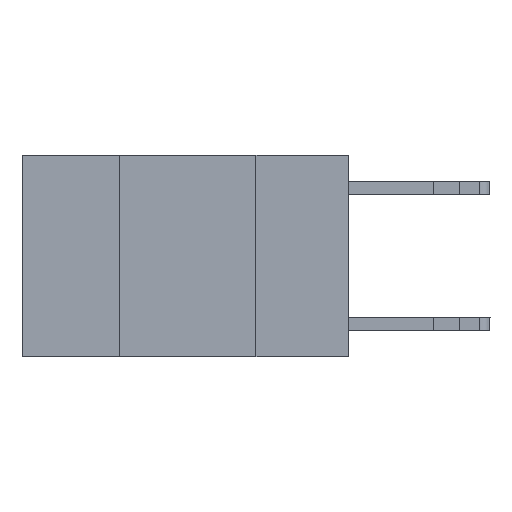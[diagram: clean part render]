
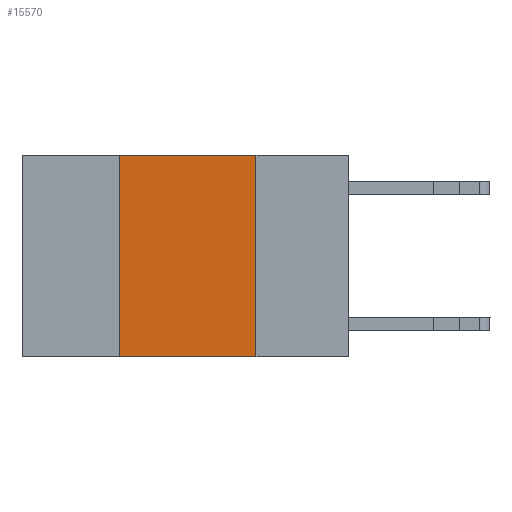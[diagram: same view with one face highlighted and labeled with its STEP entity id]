
A CAD part, left-side view. The second image highlights one B-rep face of the part: STEP entity #15570.
In plain terms, the highlighted planar face has unit normal (-1, 0, 0).
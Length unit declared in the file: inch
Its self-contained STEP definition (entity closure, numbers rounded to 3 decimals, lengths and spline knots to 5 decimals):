
#654 = ORIENTED_EDGE ( 'NONE', *, *, #1391, .F. ) ;
#1391 = EDGE_CURVE ( 'NONE', #5841, #13872, #3553, .T. ) ;
#1928 = CARTESIAN_POINT ( 'NONE',  ( 0., 0.42, 0. ) ) ;
#3122 = EDGE_CURVE ( 'NONE', #23136, #13872, #21978, .T. ) ;
#3553 = LINE ( 'NONE', #5529, #25865 ) ;
#4776 = VECTOR ( 'NONE', #12454, 39.37008 ) ;
#5529 = CARTESIAN_POINT ( 'NONE',  ( 0., 0.17, 0. ) ) ;
#5841 = VERTEX_POINT ( 'NONE', #16733 ) ;
#5998 = CARTESIAN_POINT ( 'NONE',  ( 0., 0.6, 0. ) ) ;
#7712 = CARTESIAN_POINT ( 'NONE',  ( 0., 0.6, 0. ) ) ;
#8112 = VECTOR ( 'NONE', #10567, 39.37008 ) ;
#9102 = EDGE_CURVE ( 'NONE', #23136, #19606, #25375, .T. ) ;
#10280 = DIRECTION ( 'NONE',  ( 0., 0., -1. ) ) ;
#10282 = CARTESIAN_POINT ( 'NONE',  ( 0., 0.6, -0.37 ) ) ;
#10567 = DIRECTION ( 'NONE',  ( 0., 0., 1. ) ) ;
#12454 = DIRECTION ( 'NONE',  ( 0., -1., 0. ) ) ;
#12634 = ORIENTED_EDGE ( 'NONE', *, *, #3122, .T. ) ;
#13872 = VERTEX_POINT ( 'NONE', #19781 ) ;
#14551 = VECTOR ( 'NONE', #20623, 39.37008 ) ;
#15570 = ADVANCED_FACE ( 'NONE', ( #25257 ), #27630, .F. ) ;
#16733 = CARTESIAN_POINT ( 'NONE',  ( 0., 0.17, 0. ) ) ;
#19606 = VERTEX_POINT ( 'NONE', #1928 ) ;
#19781 = CARTESIAN_POINT ( 'NONE',  ( 0., 0.17, -0.37 ) ) ;
#19862 = CARTESIAN_POINT ( 'NONE',  ( 0., 0.42, -0.37 ) ) ;
#20305 = LINE ( 'NONE', #7712, #14551 ) ;
#20623 = DIRECTION ( 'NONE',  ( 0., -1., 0. ) ) ;
#21144 = AXIS2_PLACEMENT_3D ( 'NONE', #5998, #23246, #10280 ) ;
#21352 = CARTESIAN_POINT ( 'NONE',  ( 0., 0.42, 0. ) ) ;
#21978 = LINE ( 'NONE', #10282, #4776 ) ;
#22270 = ORIENTED_EDGE ( 'NONE', *, *, #9102, .F. ) ;
#23136 = VERTEX_POINT ( 'NONE', #19862 ) ;
#23246 = DIRECTION ( 'NONE',  ( 1., 0., 0. ) ) ;
#23319 = ORIENTED_EDGE ( 'NONE', *, *, #27092, .F. ) ;
#23857 = DIRECTION ( 'NONE',  ( 0., 0., -1. ) ) ;
#23919 = EDGE_LOOP ( 'NONE', ( #654, #23319, #22270, #12634 ) ) ;
#25257 = FACE_OUTER_BOUND ( 'NONE', #23919, .T. ) ;
#25375 = LINE ( 'NONE', #21352, #8112 ) ;
#25865 = VECTOR ( 'NONE', #23857, 39.37008 ) ;
#27092 = EDGE_CURVE ( 'NONE', #19606, #5841, #20305, .T. ) ;
#27630 = PLANE ( 'NONE',  #21144 ) ;
